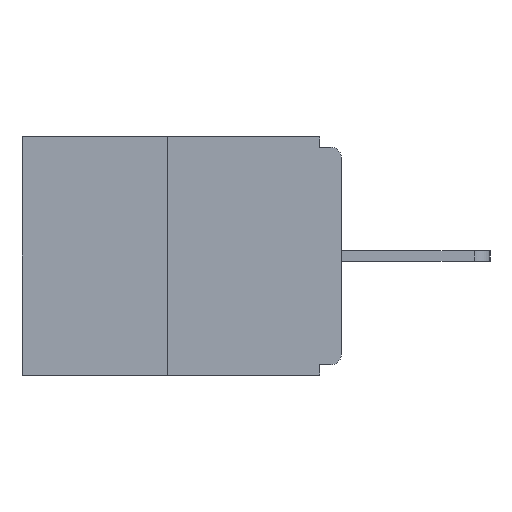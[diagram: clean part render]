
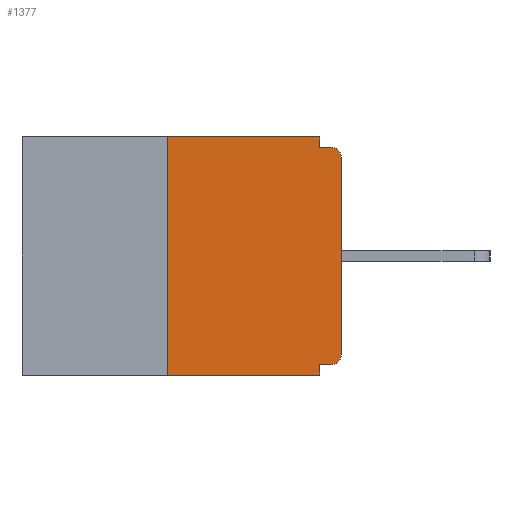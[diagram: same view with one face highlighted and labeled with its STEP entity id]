
A CAD part, left-side view. The second image highlights one B-rep face of the part: STEP entity #1377.
In plain terms, the highlighted planar face has unit normal (-1, 0, 0).
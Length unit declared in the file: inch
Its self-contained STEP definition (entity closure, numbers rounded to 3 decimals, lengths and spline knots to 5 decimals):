
#31 = DIRECTION ( 'NONE',  ( -1., 0., 0. ) ) ;
#107 = LINE ( 'NONE', #3145, #14158 ) ;
#215 = ORIENTED_EDGE ( 'NONE', *, *, #4600, .T. ) ;
#392 = CARTESIAN_POINT ( 'NONE',  ( 0., 0., -0.328 ) ) ;
#661 = ORIENTED_EDGE ( 'NONE', *, *, #1826, .F. ) ;
#720 = CARTESIAN_POINT ( 'NONE',  ( 0., 0.46, 0. ) ) ;
#772 = DIRECTION ( 'NONE',  ( 0., -1., 0. ) ) ;
#799 = EDGE_CURVE ( 'NONE', #19626, #16678, #5028, .T. ) ;
#804 = VECTOR ( 'NONE', #7157, 39.37008 ) ;
#1377 = ADVANCED_FACE ( 'NONE', ( #12764 ), #11276, .F. ) ;
#1411 = ORIENTED_EDGE ( 'NONE', *, *, #3550, .F. ) ;
#1826 = EDGE_CURVE ( 'NONE', #19626, #3328, #17135, .T. ) ;
#2044 = AXIS2_PLACEMENT_3D ( 'NONE', #16934, #13536, #3225 ) ;
#2366 = EDGE_CURVE ( 'NONE', #11815, #5718, #14496, .T. ) ;
#2704 = ORIENTED_EDGE ( 'NONE', *, *, #16639, .F. ) ;
#2973 = CARTESIAN_POINT ( 'NONE',  ( 0., 0.015, -0.313 ) ) ;
#3145 = CARTESIAN_POINT ( 'NONE',  ( 0., 0.25, 0. ) ) ;
#3146 = VERTEX_POINT ( 'NONE', #12054 ) ;
#3225 = DIRECTION ( 'NONE',  ( 0., 0., -1. ) ) ;
#3328 = VERTEX_POINT ( 'NONE', #8030 ) ;
#3550 = EDGE_CURVE ( 'NONE', #3328, #5718, #4871, .T. ) ;
#3724 = ORIENTED_EDGE ( 'NONE', *, *, #799, .T. ) ;
#3765 = CARTESIAN_POINT ( 'NONE',  ( 0., 0.25, -0.343 ) ) ;
#4033 = EDGE_CURVE ( 'NONE', #11815, #18317, #107, .T. ) ;
#4100 = ORIENTED_EDGE ( 'NONE', *, *, #15100, .T. ) ;
#4600 = EDGE_CURVE ( 'NONE', #16678, #11077, #9641, .T. ) ;
#4871 = LINE ( 'NONE', #12389, #5468 ) ;
#5028 = CIRCLE ( 'NONE', #9516, 0.015 ) ;
#5335 = DIRECTION ( 'NONE',  ( 0., 0., 1. ) ) ;
#5468 = VECTOR ( 'NONE', #9303, 39.37008 ) ;
#5718 = VERTEX_POINT ( 'NONE', #18566 ) ;
#5777 = ORIENTED_EDGE ( 'NONE', *, *, #4033, .F. ) ;
#5828 = AXIS2_PLACEMENT_3D ( 'NONE', #720, #6759, #18785 ) ;
#6260 = VECTOR ( 'NONE', #5335, 39.37008 ) ;
#6576 = EDGE_CURVE ( 'NONE', #18317, #13171, #18411, .T. ) ;
#6620 = DIRECTION ( 'NONE',  ( 0., 0., -1. ) ) ;
#6759 = DIRECTION ( 'NONE',  ( 1., 0., 0. ) ) ;
#7157 = DIRECTION ( 'NONE',  ( 0., -1., 0. ) ) ;
#8030 = CARTESIAN_POINT ( 'NONE',  ( 0., 0.031, -0.328 ) ) ;
#8297 = VECTOR ( 'NONE', #15086, 39.37008 ) ;
#8564 = CARTESIAN_POINT ( 'NONE',  ( 0., 0., -0.313 ) ) ;
#9303 = DIRECTION ( 'NONE',  ( 0., 0., -1. ) ) ;
#9483 = EDGE_LOOP ( 'NONE', ( #15462, #5777, #12119, #1411, #661, #3724, #215, #4100, #2704, #18872 ) ) ;
#9516 = AXIS2_PLACEMENT_3D ( 'NONE', #2973, #31, #16886 ) ;
#9641 = LINE ( 'NONE', #13028, #6260 ) ;
#11054 = CARTESIAN_POINT ( 'NONE',  ( 0., 0., -0.03 ) ) ;
#11077 = VERTEX_POINT ( 'NONE', #11054 ) ;
#11276 = PLANE ( 'NONE',  #5828 ) ;
#11347 = CARTESIAN_POINT ( 'NONE',  ( 0., 0.031, 0. ) ) ;
#11815 = VERTEX_POINT ( 'NONE', #3765 ) ;
#12020 = CARTESIAN_POINT ( 'NONE',  ( 0., 0.015, -0.328 ) ) ;
#12054 = CARTESIAN_POINT ( 'NONE',  ( 0., 0.031, -0.015 ) ) ;
#12119 = ORIENTED_EDGE ( 'NONE', *, *, #2366, .T. ) ;
#12389 = CARTESIAN_POINT ( 'NONE',  ( 0., 0.031, -0.343 ) ) ;
#12622 = CIRCLE ( 'NONE', #2044, 0.015 ) ;
#12631 = LINE ( 'NONE', #11347, #17046 ) ;
#12764 = FACE_OUTER_BOUND ( 'NONE', #9483, .T. ) ;
#13028 = CARTESIAN_POINT ( 'NONE',  ( 0., 0., 0. ) ) ;
#13056 = LINE ( 'NONE', #17378, #804 ) ;
#13171 = VERTEX_POINT ( 'NONE', #13181 ) ;
#13181 = CARTESIAN_POINT ( 'NONE',  ( 0., 0.031, 0. ) ) ;
#13536 = DIRECTION ( 'NONE',  ( -1., 0., 0. ) ) ;
#13925 = EDGE_CURVE ( 'NONE', #13171, #3146, #12631, .T. ) ;
#14158 = VECTOR ( 'NONE', #15356, 39.37008 ) ;
#14496 = LINE ( 'NONE', #16574, #16199 ) ;
#15086 = DIRECTION ( 'NONE',  ( 0., -1., 0. ) ) ;
#15100 = EDGE_CURVE ( 'NONE', #11077, #19397, #12622, .T. ) ;
#15356 = DIRECTION ( 'NONE',  ( 0., 0., 1. ) ) ;
#15389 = CARTESIAN_POINT ( 'NONE',  ( 0., 0.46, 0. ) ) ;
#15462 = ORIENTED_EDGE ( 'NONE', *, *, #6576, .F. ) ;
#16052 = CARTESIAN_POINT ( 'NONE',  ( 0., 0.25, 0. ) ) ;
#16199 = VECTOR ( 'NONE', #772, 39.37008 ) ;
#16574 = CARTESIAN_POINT ( 'NONE',  ( 0., 0.46, -0.343 ) ) ;
#16639 = EDGE_CURVE ( 'NONE', #3146, #19397, #13056, .T. ) ;
#16678 = VERTEX_POINT ( 'NONE', #8564 ) ;
#16886 = DIRECTION ( 'NONE',  ( 0., 0., -1. ) ) ;
#16934 = CARTESIAN_POINT ( 'NONE',  ( 0., 0.015, -0.03 ) ) ;
#17046 = VECTOR ( 'NONE', #6620, 39.37008 ) ;
#17135 = LINE ( 'NONE', #392, #19514 ) ;
#17244 = DIRECTION ( 'NONE',  ( 0., 1., 0. ) ) ;
#17378 = CARTESIAN_POINT ( 'NONE',  ( 0., 0., -0.015 ) ) ;
#17734 = CARTESIAN_POINT ( 'NONE',  ( 0., 0.015, -0.015 ) ) ;
#18317 = VERTEX_POINT ( 'NONE', #16052 ) ;
#18411 = LINE ( 'NONE', #15389, #8297 ) ;
#18566 = CARTESIAN_POINT ( 'NONE',  ( 0., 0.031, -0.343 ) ) ;
#18785 = DIRECTION ( 'NONE',  ( 0., 0., -1. ) ) ;
#18872 = ORIENTED_EDGE ( 'NONE', *, *, #13925, .F. ) ;
#19397 = VERTEX_POINT ( 'NONE', #17734 ) ;
#19514 = VECTOR ( 'NONE', #17244, 39.37008 ) ;
#19626 = VERTEX_POINT ( 'NONE', #12020 ) ;
